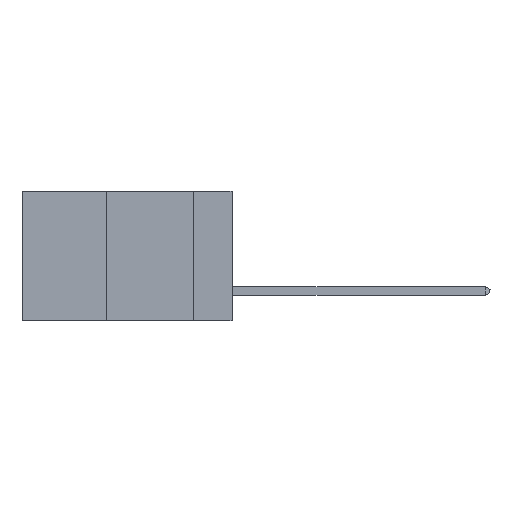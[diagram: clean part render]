
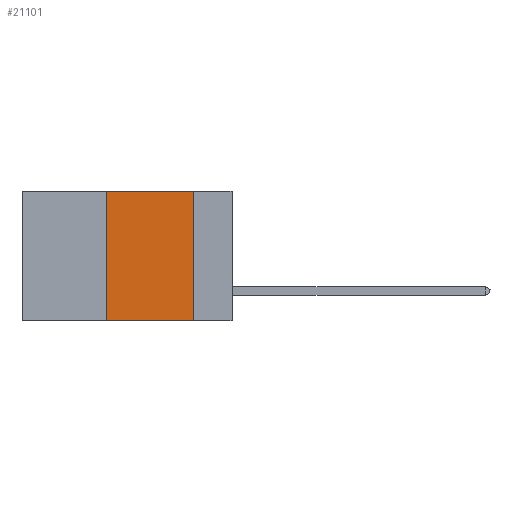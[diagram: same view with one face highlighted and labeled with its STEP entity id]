
A CAD part, left-side view. The second image highlights one B-rep face of the part: STEP entity #21101.
In plain terms, the highlighted planar face has unit normal (-1, 0, 0).
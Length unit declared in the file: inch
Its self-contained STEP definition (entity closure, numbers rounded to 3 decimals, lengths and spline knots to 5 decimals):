
#2962 = EDGE_LOOP ( 'NONE', ( #42645, #47530, #3982, #29815 ) ) ;
#3356 = VECTOR ( 'NONE', #42373, 39.37008 ) ;
#3982 = ORIENTED_EDGE ( 'NONE', *, *, #10342, .F. ) ;
#6139 = CARTESIAN_POINT ( 'NONE',  ( 0., 0.36, 0. ) ) ;
#7378 = EDGE_CURVE ( 'NONE', #12257, #43060, #21918, .T. ) ;
#9321 = CARTESIAN_POINT ( 'NONE',  ( 0., 0.11, -0.37 ) ) ;
#10342 = EDGE_CURVE ( 'NONE', #41193, #12257, #36520, .T. ) ;
#12257 = VERTEX_POINT ( 'NONE', #47077 ) ;
#12860 = EDGE_CURVE ( 'NONE', #43060, #24550, #48400, .T. ) ;
#13577 = DIRECTION ( 'NONE',  ( 0., -1., 0. ) ) ;
#14409 = VECTOR ( 'NONE', #32996, 39.37008 ) ;
#15919 = CARTESIAN_POINT ( 'NONE',  ( 0., 0.36, -0.37 ) ) ;
#16331 = DIRECTION ( 'NONE',  ( 1., 0., 0. ) ) ;
#17610 = CARTESIAN_POINT ( 'NONE',  ( 0., 0.11, 0. ) ) ;
#20509 = CARTESIAN_POINT ( 'NONE',  ( 0., 0.11, 0. ) ) ;
#21101 = ADVANCED_FACE ( 'NONE', ( #33806 ), #28236, .F. ) ;
#21918 = LINE ( 'NONE', #34041, #41153 ) ;
#24550 = VERTEX_POINT ( 'NONE', #9321 ) ;
#27872 = VECTOR ( 'NONE', #40191, 39.37008 ) ;
#28236 = PLANE ( 'NONE',  #39550 ) ;
#29815 = ORIENTED_EDGE ( 'NONE', *, *, #41801, .T. ) ;
#30738 = CARTESIAN_POINT ( 'NONE',  ( 0., 0.6, -0.37 ) ) ;
#32996 = DIRECTION ( 'NONE',  ( 0., 0., 1. ) ) ;
#33317 = LINE ( 'NONE', #30738, #3356 ) ;
#33806 = FACE_OUTER_BOUND ( 'NONE', #2962, .T. ) ;
#34041 = CARTESIAN_POINT ( 'NONE',  ( 0., 0.6, 0. ) ) ;
#36520 = LINE ( 'NONE', #6139, #14409 ) ;
#39309 = CARTESIAN_POINT ( 'NONE',  ( 0., 0.6, 0. ) ) ;
#39550 = AXIS2_PLACEMENT_3D ( 'NONE', #39309, #16331, #43134 ) ;
#40191 = DIRECTION ( 'NONE',  ( 0., 0., -1. ) ) ;
#41153 = VECTOR ( 'NONE', #13577, 39.37008 ) ;
#41193 = VERTEX_POINT ( 'NONE', #15919 ) ;
#41801 = EDGE_CURVE ( 'NONE', #41193, #24550, #33317, .T. ) ;
#42373 = DIRECTION ( 'NONE',  ( 0., -1., 0. ) ) ;
#42645 = ORIENTED_EDGE ( 'NONE', *, *, #12860, .F. ) ;
#43060 = VERTEX_POINT ( 'NONE', #20509 ) ;
#43134 = DIRECTION ( 'NONE',  ( 0., 0., -1. ) ) ;
#47077 = CARTESIAN_POINT ( 'NONE',  ( 0., 0.36, 0. ) ) ;
#47530 = ORIENTED_EDGE ( 'NONE', *, *, #7378, .F. ) ;
#48400 = LINE ( 'NONE', #17610, #27872 ) ;
